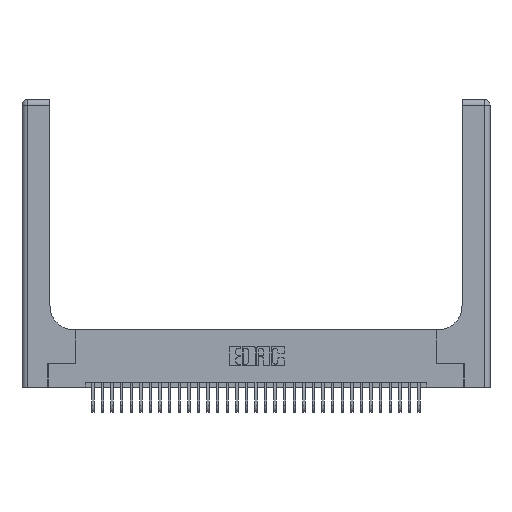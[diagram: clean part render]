
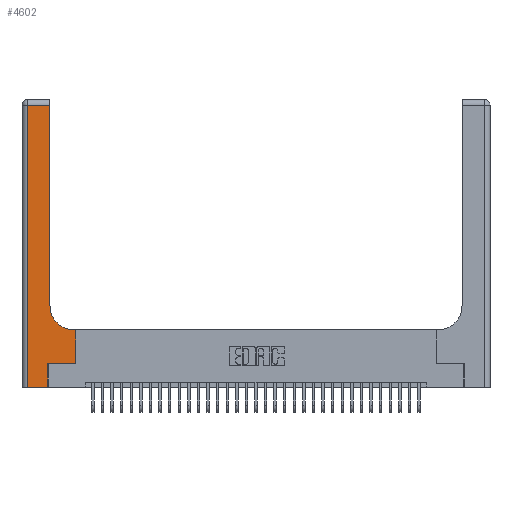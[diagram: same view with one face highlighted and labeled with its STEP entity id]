
A CAD part, top view. The second image highlights one B-rep face of the part: STEP entity #4602.
In plain terms, the highlighted planar face has unit normal (0, 0, 1).
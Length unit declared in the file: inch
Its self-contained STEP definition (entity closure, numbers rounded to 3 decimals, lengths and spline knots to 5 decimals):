
#394 = VERTEX_POINT ( 'NONE', #32436 ) ;
#402 = LINE ( 'NONE', #10985, #6473 ) ;
#737 = VECTOR ( 'NONE', #16567, 39.37008 ) ;
#1217 = PLANE ( 'NONE',  #10855 ) ;
#1403 = EDGE_CURVE ( 'NONE', #26138, #3391, #7642, .T. ) ;
#1754 = FACE_OUTER_BOUND ( 'NONE', #4325, .T. ) ;
#2556 = ORIENTED_EDGE ( 'NONE', *, *, #21373, .T. ) ;
#2575 = CARTESIAN_POINT ( 'NONE',  ( 0.06, 2.94, 0.37 ) ) ;
#3391 = VERTEX_POINT ( 'NONE', #26643 ) ;
#3620 = VERTEX_POINT ( 'NONE', #14942 ) ;
#3842 = DIRECTION ( 'NONE',  ( -1., 0., 0. ) ) ;
#4121 = DIRECTION ( 'NONE',  ( -1., 0., 0. ) ) ;
#4325 = EDGE_LOOP ( 'NONE', ( #2556, #27358, #14702, #20194, #9732, #21068, #6402, #23603, #23042 ) ) ;
#4471 = VERTEX_POINT ( 'NONE', #15740 ) ;
#4602 = ADVANCED_FACE ( 'NONE', ( #1754 ), #1217, .F. ) ;
#4720 = DIRECTION ( 'NONE',  ( 0., 1., 0. ) ) ;
#5335 = CARTESIAN_POINT ( 'NONE',  ( 0.06, 3., 0.37 ) ) ;
#5645 = LINE ( 'NONE', #7169, #12412 ) ;
#6167 = VECTOR ( 'NONE', #27940, 39.37008 ) ;
#6327 = CARTESIAN_POINT ( 'NONE',  ( 0., 3., 0.37 ) ) ;
#6402 = ORIENTED_EDGE ( 'NONE', *, *, #23685, .T. ) ;
#6473 = VECTOR ( 'NONE', #28524, 39.37008 ) ;
#6611 = VERTEX_POINT ( 'NONE', #26651 ) ;
#6841 = VECTOR ( 'NONE', #7889, 39.37008 ) ;
#7169 = CARTESIAN_POINT ( 'NONE',  ( 0.2915, 3., 0.37 ) ) ;
#7642 = LINE ( 'NONE', #13737, #13606 ) ;
#7889 = DIRECTION ( 'NONE',  ( 0., -1., 0. ) ) ;
#8401 = LINE ( 'NONE', #14071, #737 ) ;
#8772 = EDGE_CURVE ( 'NONE', #394, #16690, #27684, .T. ) ;
#9410 = DIRECTION ( 'NONE',  ( 0., 0., -1. ) ) ;
#9422 = CARTESIAN_POINT ( 'NONE',  ( 0.269, 0.25, 0.37 ) ) ;
#9732 = ORIENTED_EDGE ( 'NONE', *, *, #30796, .T. ) ;
#10311 = VECTOR ( 'NONE', #27027, 39.37008 ) ;
#10528 = EDGE_CURVE ( 'NONE', #16052, #394, #26783, .T. ) ;
#10854 = CARTESIAN_POINT ( 'NONE',  ( 0.2915, 0.85, 0.37 ) ) ;
#10855 = AXIS2_PLACEMENT_3D ( 'NONE', #6327, #18984, #3842 ) ;
#10985 = CARTESIAN_POINT ( 'NONE',  ( 0.269, 0., 0.37 ) ) ;
#11913 = CARTESIAN_POINT ( 'NONE',  ( 0.5585, 0.25, 0.37 ) ) ;
#12412 = VECTOR ( 'NONE', #4720, 39.37008 ) ;
#13606 = VECTOR ( 'NONE', #28594, 39.37008 ) ;
#13737 = CARTESIAN_POINT ( 'NONE',  ( 0.269, 0.25, 0.37 ) ) ;
#14071 = CARTESIAN_POINT ( 'NONE',  ( 0.2915, 0.6, 0.37 ) ) ;
#14251 = CARTESIAN_POINT ( 'NONE',  ( 0., 2.94, 0.37 ) ) ;
#14702 = ORIENTED_EDGE ( 'NONE', *, *, #10528, .T. ) ;
#14942 = CARTESIAN_POINT ( 'NONE',  ( 0.5585, 0.6, 0.37 ) ) ;
#15451 = CARTESIAN_POINT ( 'NONE',  ( 0.269, 0., 0.37 ) ) ;
#15740 = CARTESIAN_POINT ( 'NONE',  ( 0.5415, 0.6, 0.37 ) ) ;
#16052 = VERTEX_POINT ( 'NONE', #2575 ) ;
#16326 = CIRCLE ( 'NONE', #21630, 0.25 ) ;
#16567 = DIRECTION ( 'NONE',  ( -1., 0., 0. ) ) ;
#16632 = VECTOR ( 'NONE', #4121, 39.37008 ) ;
#16690 = VERTEX_POINT ( 'NONE', #15451 ) ;
#17436 = LINE ( 'NONE', #14251, #16632 ) ;
#18984 = DIRECTION ( 'NONE',  ( 0., 0., -1. ) ) ;
#19434 = VERTEX_POINT ( 'NONE', #10854 ) ;
#20194 = ORIENTED_EDGE ( 'NONE', *, *, #8772, .T. ) ;
#21068 = ORIENTED_EDGE ( 'NONE', *, *, #1403, .T. ) ;
#21249 = EDGE_CURVE ( 'NONE', #4471, #19434, #16326, .T. ) ;
#21373 = EDGE_CURVE ( 'NONE', #19434, #6611, #5645, .T. ) ;
#21630 = AXIS2_PLACEMENT_3D ( 'NONE', #24369, #9410, #26855 ) ;
#22762 = CARTESIAN_POINT ( 'NONE',  ( 0., 0., 0.37 ) ) ;
#23042 = ORIENTED_EDGE ( 'NONE', *, *, #21249, .T. ) ;
#23595 = LINE ( 'NONE', #11913, #10311 ) ;
#23603 = ORIENTED_EDGE ( 'NONE', *, *, #28259, .T. ) ;
#23685 = EDGE_CURVE ( 'NONE', #3391, #3620, #23595, .T. ) ;
#24369 = CARTESIAN_POINT ( 'NONE',  ( 0.5415, 0.85, 0.37 ) ) ;
#26138 = VERTEX_POINT ( 'NONE', #9422 ) ;
#26643 = CARTESIAN_POINT ( 'NONE',  ( 0.5585, 0.25, 0.37 ) ) ;
#26651 = CARTESIAN_POINT ( 'NONE',  ( 0.2915, 2.94, 0.37 ) ) ;
#26783 = LINE ( 'NONE', #5335, #6841 ) ;
#26855 = DIRECTION ( 'NONE',  ( 1., 0., 0. ) ) ;
#27027 = DIRECTION ( 'NONE',  ( 0., 1., 0. ) ) ;
#27358 = ORIENTED_EDGE ( 'NONE', *, *, #32181, .T. ) ;
#27684 = LINE ( 'NONE', #22762, #6167 ) ;
#27940 = DIRECTION ( 'NONE',  ( 1., 0., 0. ) ) ;
#28259 = EDGE_CURVE ( 'NONE', #3620, #4471, #8401, .T. ) ;
#28524 = DIRECTION ( 'NONE',  ( 0., 1., 0. ) ) ;
#28594 = DIRECTION ( 'NONE',  ( 1., 0., 0. ) ) ;
#30796 = EDGE_CURVE ( 'NONE', #16690, #26138, #402, .T. ) ;
#32181 = EDGE_CURVE ( 'NONE', #6611, #16052, #17436, .T. ) ;
#32436 = CARTESIAN_POINT ( 'NONE',  ( 0.06, 0., 0.37 ) ) ;
